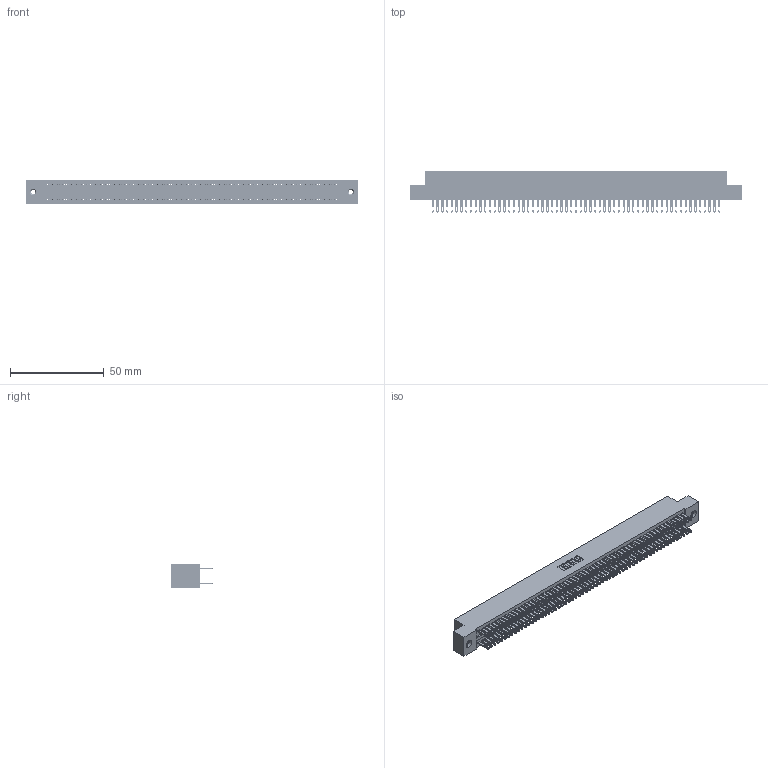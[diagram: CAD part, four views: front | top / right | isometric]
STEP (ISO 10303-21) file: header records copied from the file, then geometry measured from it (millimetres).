
FILE_DESCRIPTION (( 'STEP AP203' ), '1' );
FILE_NAME ('325-122-500-208.STEP', '2020-02-25T08:52:39', ( '' ), ( '' ), 'SwSTEP 2.0', 'SolidWorks 2016', '' );
FILE_SCHEMA (( 'CONFIG_CONTROL_DESIGN' ));
Length unit declared in the file: inch
Products named in the file (4): 325-122-500-208; 345-250-001_345-250-003-102; 325-292-001_325-293-100; 325 Part_TI
Assembly tree (125 placements, depth 2):
  325-122-500-208
    325 Part_TI
    325-292-001_325-293-100  x122
    345-250-001_345-250-003-102  x2
Bounding box: 176.66 x 21.84 x 12.45 mm (x, y, z)
Volume: 23342.5 mm3; surface area: 29992.8 mm2
Topology: 125 solids, 125 shells, 6030 faces, 18381 edges, 12246 vertices
Faces by surface type: plane 3762, cylinder 2252, cone 12, torus 4
Entity records: 37902 total; most frequent: CARTESIAN_POINT 6241, ORIENTED_EDGE 6170, DIRECTION 5331, EDGE_CURVE 3085, LINE 2933, VECTOR 2933, VERTEX_POINT 2052, AXIS2_PLACEMENT_3D 1199
